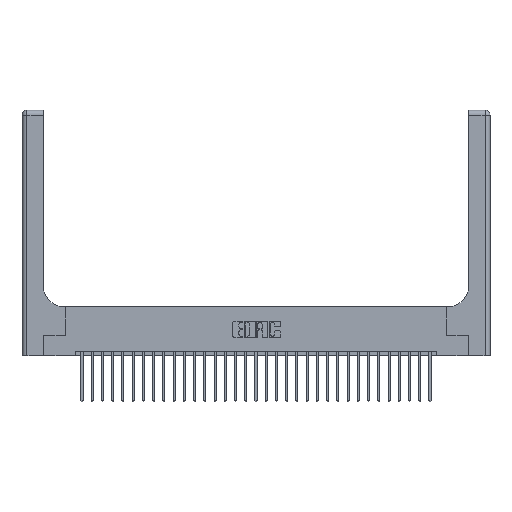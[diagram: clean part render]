
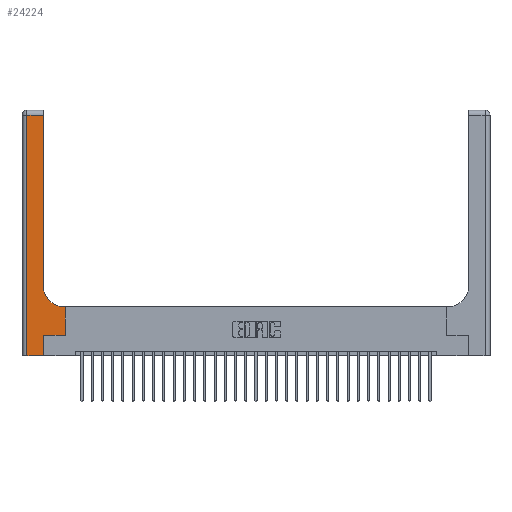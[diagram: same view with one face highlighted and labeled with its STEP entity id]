
A CAD part, top view. The second image highlights one B-rep face of the part: STEP entity #24224.
In plain terms, the highlighted planar face has unit normal (0, 0, 1).
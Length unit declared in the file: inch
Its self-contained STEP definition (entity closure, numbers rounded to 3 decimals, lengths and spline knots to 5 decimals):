
#1873 = CARTESIAN_POINT ( 'NONE',  ( 0.51, 0.85, 0.37 ) ) ;
#2571 = CARTESIAN_POINT ( 'NONE',  ( 0., 2.94, 0.37 ) ) ;
#2989 = VERTEX_POINT ( 'NONE', #12569 ) ;
#3162 = EDGE_LOOP ( 'NONE', ( #20656, #14257, #29042, #12807, #17542, #25574, #16072, #28515, #4052 ) ) ;
#3264 = EDGE_CURVE ( 'NONE', #28134, #24680, #23698, .T. ) ;
#3619 = CARTESIAN_POINT ( 'NONE',  ( 0.26, 0.85, 0.37 ) ) ;
#4052 = ORIENTED_EDGE ( 'NONE', *, *, #18200, .T. ) ;
#4694 = LINE ( 'NONE', #16008, #5207 ) ;
#4779 = VECTOR ( 'NONE', #17555, 39.37008 ) ;
#5207 = VECTOR ( 'NONE', #25249, 39.37008 ) ;
#5236 = CARTESIAN_POINT ( 'NONE',  ( 0.51, 0.6, 0.37 ) ) ;
#7365 = LINE ( 'NONE', #25543, #28938 ) ;
#8102 = CARTESIAN_POINT ( 'NONE',  ( 0.265, 0., 0.37 ) ) ;
#8834 = DIRECTION ( 'NONE',  ( 1., 0., 0. ) ) ;
#9152 = EDGE_CURVE ( 'NONE', #2989, #27886, #7365, .T. ) ;
#9240 = EDGE_CURVE ( 'NONE', #24680, #2989, #4694, .T. ) ;
#9360 = VECTOR ( 'NONE', #18864, 39.37008 ) ;
#10487 = DIRECTION ( 'NONE',  ( -1., 0., 0. ) ) ;
#10973 = VECTOR ( 'NONE', #21465, 39.37008 ) ;
#11126 = CARTESIAN_POINT ( 'NONE',  ( 0.528, 0.6, 0.37 ) ) ;
#11569 = DIRECTION ( 'NONE',  ( 0., 0., -1. ) ) ;
#11615 = CARTESIAN_POINT ( 'NONE',  ( 0.06, 2.94, 0.37 ) ) ;
#11987 = CARTESIAN_POINT ( 'NONE',  ( 0.265, 0., 0.37 ) ) ;
#12165 = CARTESIAN_POINT ( 'NONE',  ( 0.06, 3., 0.37 ) ) ;
#12569 = CARTESIAN_POINT ( 'NONE',  ( 0.528, 0.25, 0.37 ) ) ;
#12807 = ORIENTED_EDGE ( 'NONE', *, *, #23024, .T. ) ;
#12966 = LINE ( 'NONE', #20137, #18740 ) ;
#13053 = LINE ( 'NONE', #2571, #14421 ) ;
#13382 = CARTESIAN_POINT ( 'NONE',  ( 0.26, 3., 0.37 ) ) ;
#14208 = DIRECTION ( 'NONE',  ( 0., 1., 0. ) ) ;
#14257 = ORIENTED_EDGE ( 'NONE', *, *, #24024, .T. ) ;
#14421 = VECTOR ( 'NONE', #16293, 39.37008 ) ;
#14576 = AXIS2_PLACEMENT_3D ( 'NONE', #1873, #11569, #17979 ) ;
#15532 = CARTESIAN_POINT ( 'NONE',  ( 0.06, 0., 0.37 ) ) ;
#16008 = CARTESIAN_POINT ( 'NONE',  ( 0.265, 0.25, 0.37 ) ) ;
#16072 = ORIENTED_EDGE ( 'NONE', *, *, #9152, .T. ) ;
#16293 = DIRECTION ( 'NONE',  ( -1., 0., 0. ) ) ;
#16488 = AXIS2_PLACEMENT_3D ( 'NONE', #25975, #21769, #10487 ) ;
#17542 = ORIENTED_EDGE ( 'NONE', *, *, #3264, .T. ) ;
#17555 = DIRECTION ( 'NONE',  ( 0., 1., 0. ) ) ;
#17979 = DIRECTION ( 'NONE',  ( 1., 0., 0. ) ) ;
#18200 = EDGE_CURVE ( 'NONE', #23343, #19795, #19815, .T. ) ;
#18740 = VECTOR ( 'NONE', #8834, 39.37008 ) ;
#18864 = DIRECTION ( 'NONE',  ( 0., -1., 0. ) ) ;
#19112 = LINE ( 'NONE', #25668, #10973 ) ;
#19795 = VERTEX_POINT ( 'NONE', #3619 ) ;
#19815 = CIRCLE ( 'NONE', #14576, 0.25 ) ;
#20102 = CARTESIAN_POINT ( 'NONE',  ( 0.26, 2.94, 0.37 ) ) ;
#20137 = CARTESIAN_POINT ( 'NONE',  ( 0., 0., 0.37 ) ) ;
#20656 = ORIENTED_EDGE ( 'NONE', *, *, #20659, .T. ) ;
#20659 = EDGE_CURVE ( 'NONE', #19795, #23406, #26655, .T. ) ;
#21206 = VERTEX_POINT ( 'NONE', #15532 ) ;
#21340 = FACE_OUTER_BOUND ( 'NONE', #3162, .T. ) ;
#21465 = DIRECTION ( 'NONE',  ( -1., 0., 0. ) ) ;
#21587 = EDGE_CURVE ( 'NONE', #27886, #23343, #19112, .T. ) ;
#21769 = DIRECTION ( 'NONE',  ( 0., 0., -1. ) ) ;
#23024 = EDGE_CURVE ( 'NONE', #21206, #28134, #12966, .T. ) ;
#23307 = LINE ( 'NONE', #12165, #9360 ) ;
#23343 = VERTEX_POINT ( 'NONE', #5236 ) ;
#23406 = VERTEX_POINT ( 'NONE', #20102 ) ;
#23662 = VERTEX_POINT ( 'NONE', #11615 ) ;
#23698 = LINE ( 'NONE', #11987, #26606 ) ;
#24024 = EDGE_CURVE ( 'NONE', #23406, #23662, #13053, .T. ) ;
#24224 = ADVANCED_FACE ( 'NONE', ( #21340 ), #28769, .F. ) ;
#24680 = VERTEX_POINT ( 'NONE', #26366 ) ;
#25249 = DIRECTION ( 'NONE',  ( 1., 0., 0. ) ) ;
#25543 = CARTESIAN_POINT ( 'NONE',  ( 0.528, 0.25, 0.37 ) ) ;
#25574 = ORIENTED_EDGE ( 'NONE', *, *, #9240, .T. ) ;
#25668 = CARTESIAN_POINT ( 'NONE',  ( 0.26, 0.6, 0.37 ) ) ;
#25975 = CARTESIAN_POINT ( 'NONE',  ( 0., 3., 0.37 ) ) ;
#26262 = EDGE_CURVE ( 'NONE', #23662, #21206, #23307, .T. ) ;
#26366 = CARTESIAN_POINT ( 'NONE',  ( 0.265, 0.25, 0.37 ) ) ;
#26606 = VECTOR ( 'NONE', #27774, 39.37008 ) ;
#26655 = LINE ( 'NONE', #13382, #4779 ) ;
#27774 = DIRECTION ( 'NONE',  ( 0., 1., 0. ) ) ;
#27886 = VERTEX_POINT ( 'NONE', #11126 ) ;
#28134 = VERTEX_POINT ( 'NONE', #8102 ) ;
#28515 = ORIENTED_EDGE ( 'NONE', *, *, #21587, .T. ) ;
#28769 = PLANE ( 'NONE',  #16488 ) ;
#28938 = VECTOR ( 'NONE', #14208, 39.37008 ) ;
#29042 = ORIENTED_EDGE ( 'NONE', *, *, #26262, .T. ) ;
